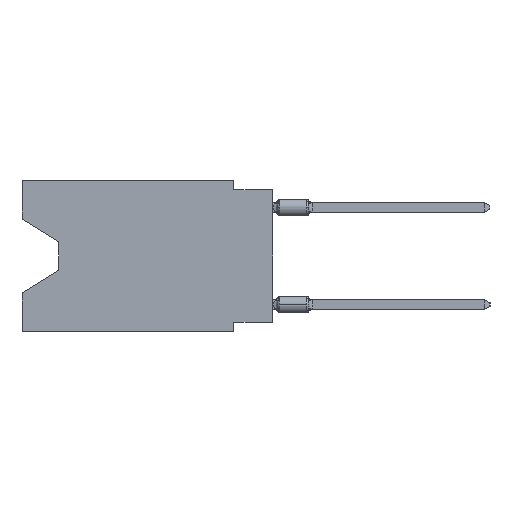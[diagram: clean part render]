
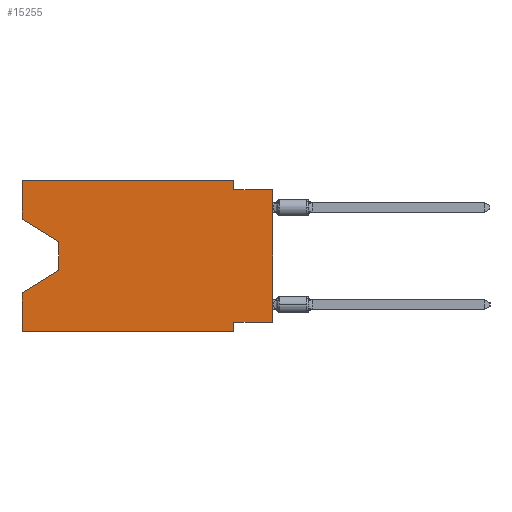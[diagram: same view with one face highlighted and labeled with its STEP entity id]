
A CAD part, left-side view. The second image highlights one B-rep face of the part: STEP entity #15255.
In plain terms, the highlighted planar face has unit normal (-1, 0, 0).
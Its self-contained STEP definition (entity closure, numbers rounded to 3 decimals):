
#530 = DIRECTION ( 'NONE',  ( 0., 0., 1. ) ) ;
#799 = VERTEX_POINT ( 'NONE', #9910 ) ;
#1073 = DIRECTION ( 'NONE',  ( 0., 0., -1. ) ) ;
#1866 = VERTEX_POINT ( 'NONE', #41592 ) ;
#2044 = CARTESIAN_POINT ( 'NONE',  ( 0., 0., -9.271 ) ) ;
#2534 = DIRECTION ( 'NONE',  ( 0., -1., 0. ) ) ;
#3008 = EDGE_CURVE ( 'NONE', #29896, #41326, #44269, .T. ) ;
#3666 = ORIENTED_EDGE ( 'NONE', *, *, #3008, .T. ) ;
#3891 = VERTEX_POINT ( 'NONE', #12305 ) ;
#3923 = CARTESIAN_POINT ( 'NONE',  ( 0., 16.383, 0. ) ) ;
#4191 = ORIENTED_EDGE ( 'NONE', *, *, #34908, .F. ) ;
#4857 = LINE ( 'NONE', #34743, #20128 ) ;
#5444 = LINE ( 'NONE', #2044, #27988 ) ;
#5890 = VECTOR ( 'NONE', #42061, 1000. ) ;
#7113 = DIRECTION ( 'NONE',  ( 0., -1., 0. ) ) ;
#7174 = ORIENTED_EDGE ( 'NONE', *, *, #46271, .T. ) ;
#8365 = EDGE_CURVE ( 'NONE', #1866, #38880, #20127, .T. ) ;
#8371 = AXIS2_PLACEMENT_3D ( 'NONE', #18094, #47735, #10804 ) ;
#8416 = ORIENTED_EDGE ( 'NONE', *, *, #35972, .T. ) ;
#9486 = VECTOR ( 'NONE', #2534, 1000. ) ;
#9910 = CARTESIAN_POINT ( 'NONE',  ( 0., 13.97, -4.013 ) ) ;
#10725 = CARTESIAN_POINT ( 'NONE',  ( 0., 2.54, -9.906 ) ) ;
#10804 = DIRECTION ( 'NONE',  ( 0., 0., -1. ) ) ;
#10925 = VERTEX_POINT ( 'NONE', #24083 ) ;
#11039 = PLANE ( 'NONE',  #8371 ) ;
#11202 = CARTESIAN_POINT ( 'NONE',  ( 0., 13.97, -4.013 ) ) ;
#12123 = DIRECTION ( 'NONE',  ( 0., 0., 1. ) ) ;
#12305 = CARTESIAN_POINT ( 'NONE',  ( 0., 13.97, -5.893 ) ) ;
#14005 = VERTEX_POINT ( 'NONE', #43287 ) ;
#15140 = VECTOR ( 'NONE', #530, 1000. ) ;
#15255 = ADVANCED_FACE ( 'NONE', ( #37041 ), #11039, .F. ) ;
#15625 = CARTESIAN_POINT ( 'NONE',  ( 0., 16.383, -9.906 ) ) ;
#17995 = EDGE_CURVE ( 'NONE', #10925, #36498, #19471, .T. ) ;
#18001 = ORIENTED_EDGE ( 'NONE', *, *, #47430, .T. ) ;
#18094 = CARTESIAN_POINT ( 'NONE',  ( 0., 16.383, 0. ) ) ;
#18803 = ORIENTED_EDGE ( 'NONE', *, *, #41468, .F. ) ;
#19471 = LINE ( 'NONE', #33830, #5890 ) ;
#20080 = DIRECTION ( 'NONE',  ( 0., -0.855, -0.519 ) ) ;
#20127 = LINE ( 'NONE', #41522, #25162 ) ;
#20128 = VECTOR ( 'NONE', #26260, 1000. ) ;
#21063 = CARTESIAN_POINT ( 'NONE',  ( 0., 16.383, -7.36 ) ) ;
#21195 = CARTESIAN_POINT ( 'NONE',  ( 0., 16.383, -2.546 ) ) ;
#21238 = DIRECTION ( 'NONE',  ( 0., 1., 0. ) ) ;
#21506 = CARTESIAN_POINT ( 'NONE',  ( 0., 0., -0.635 ) ) ;
#21913 = LINE ( 'NONE', #36474, #41892 ) ;
#22475 = LINE ( 'NONE', #30484, #33397 ) ;
#22992 = ORIENTED_EDGE ( 'NONE', *, *, #30312, .F. ) ;
#24083 = CARTESIAN_POINT ( 'NONE',  ( 0., 2.54, 0. ) ) ;
#24748 = CARTESIAN_POINT ( 'NONE',  ( 0., 16.383, 0. ) ) ;
#25114 = ORIENTED_EDGE ( 'NONE', *, *, #17995, .F. ) ;
#25162 = VECTOR ( 'NONE', #12123, 1000. ) ;
#25549 = DIRECTION ( 'NONE',  ( 0., 0.855, -0.519 ) ) ;
#26042 = LINE ( 'NONE', #3923, #15140 ) ;
#26260 = DIRECTION ( 'NONE',  ( 0., -1., 0. ) ) ;
#26345 = ORIENTED_EDGE ( 'NONE', *, *, #41494, .F. ) ;
#27988 = VECTOR ( 'NONE', #21238, 1000. ) ;
#29025 = LINE ( 'NONE', #21506, #9486 ) ;
#29202 = LINE ( 'NONE', #11202, #32674 ) ;
#29429 = DIRECTION ( 'NONE',  ( 0., 0., -1. ) ) ;
#29896 = VERTEX_POINT ( 'NONE', #15625 ) ;
#30312 = EDGE_CURVE ( 'NONE', #29896, #43173, #26042, .T. ) ;
#30484 = CARTESIAN_POINT ( 'NONE',  ( 0., 2.54, -9.906 ) ) ;
#32176 = EDGE_LOOP ( 'NONE', ( #8416, #7174, #18001, #22992, #3666, #4191, #38382, #35024, #39869, #25114, #18803, #26345 ) ) ;
#32587 = CARTESIAN_POINT ( 'NONE',  ( 0., 16.383, 0. ) ) ;
#32674 = VECTOR ( 'NONE', #29429, 1000. ) ;
#33397 = VECTOR ( 'NONE', #1073, 1000. ) ;
#33830 = CARTESIAN_POINT ( 'NONE',  ( 0., 2.54, 0. ) ) ;
#34743 = CARTESIAN_POINT ( 'NONE',  ( 0., 16.383, 0. ) ) ;
#34908 = EDGE_CURVE ( 'NONE', #14005, #41326, #22475, .T. ) ;
#35024 = ORIENTED_EDGE ( 'NONE', *, *, #8365, .T. ) ;
#35614 = LINE ( 'NONE', #35849, #41232 ) ;
#35849 = CARTESIAN_POINT ( 'NONE',  ( 0., 16.383, -2.546 ) ) ;
#35972 = EDGE_CURVE ( 'NONE', #44167, #799, #35614, .T. ) ;
#36400 = VECTOR ( 'NONE', #39564, 1000. ) ;
#36474 = CARTESIAN_POINT ( 'NONE',  ( 0., 13.97, -5.893 ) ) ;
#36498 = VERTEX_POINT ( 'NONE', #43325 ) ;
#37041 = FACE_OUTER_BOUND ( 'NONE', #32176, .T. ) ;
#38382 = ORIENTED_EDGE ( 'NONE', *, *, #45675, .F. ) ;
#38707 = EDGE_CURVE ( 'NONE', #36498, #38880, #29025, .T. ) ;
#38880 = VERTEX_POINT ( 'NONE', #41141 ) ;
#39344 = LINE ( 'NONE', #24748, #36400 ) ;
#39564 = DIRECTION ( 'NONE',  ( 0., 0., 1. ) ) ;
#39869 = ORIENTED_EDGE ( 'NONE', *, *, #38707, .F. ) ;
#40393 = CARTESIAN_POINT ( 'NONE',  ( 0., 16.383, -9.906 ) ) ;
#41141 = CARTESIAN_POINT ( 'NONE',  ( 0., 0., -0.635 ) ) ;
#41232 = VECTOR ( 'NONE', #20080, 1000. ) ;
#41326 = VERTEX_POINT ( 'NONE', #10725 ) ;
#41468 = EDGE_CURVE ( 'NONE', #47552, #10925, #4857, .T. ) ;
#41494 = EDGE_CURVE ( 'NONE', #44167, #47552, #39344, .T. ) ;
#41522 = CARTESIAN_POINT ( 'NONE',  ( 0., 0., 0. ) ) ;
#41592 = CARTESIAN_POINT ( 'NONE',  ( 0., 0., -9.271 ) ) ;
#41892 = VECTOR ( 'NONE', #25549, 1000. ) ;
#42061 = DIRECTION ( 'NONE',  ( 0., 0., -1. ) ) ;
#42274 = VECTOR ( 'NONE', #7113, 1000. ) ;
#43173 = VERTEX_POINT ( 'NONE', #21063 ) ;
#43287 = CARTESIAN_POINT ( 'NONE',  ( 0., 2.54, -9.271 ) ) ;
#43325 = CARTESIAN_POINT ( 'NONE',  ( 0., 2.54, -0.635 ) ) ;
#44167 = VERTEX_POINT ( 'NONE', #21195 ) ;
#44269 = LINE ( 'NONE', #40393, #42274 ) ;
#45675 = EDGE_CURVE ( 'NONE', #1866, #14005, #5444, .T. ) ;
#46271 = EDGE_CURVE ( 'NONE', #799, #3891, #29202, .T. ) ;
#47430 = EDGE_CURVE ( 'NONE', #3891, #43173, #21913, .T. ) ;
#47552 = VERTEX_POINT ( 'NONE', #32587 ) ;
#47735 = DIRECTION ( 'NONE',  ( 1., 0., 0. ) ) ;
